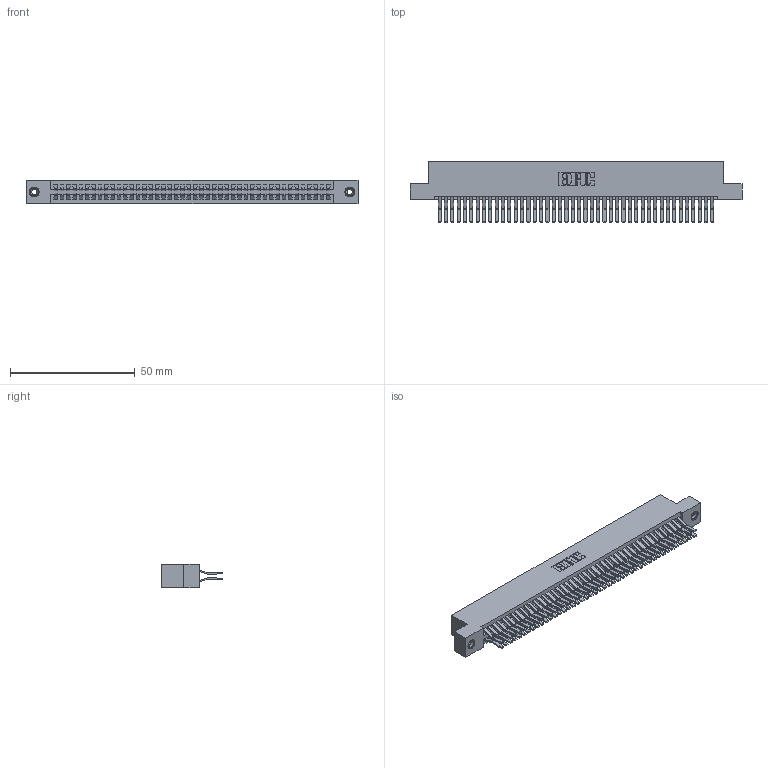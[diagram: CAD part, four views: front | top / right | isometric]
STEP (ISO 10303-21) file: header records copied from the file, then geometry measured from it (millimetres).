
FILE_DESCRIPTION (( 'STEP AP203' ), '1' );
FILE_NAME ('395-088-560-208.STEP', '2019-10-25T15:27:44', ( '' ), ( '' ), 'SwSTEP 2.0', 'SolidWorks 2016', '' );
FILE_SCHEMA (( 'CONFIG_CONTROL_DESIGN' ));
Length unit declared in the file: inch
Products named in the file (4): 345 Part_Flush Mounting Lugs - 0.156 Dia-TI; 345-292-001_560 Tail; 345-250-001_345-250-003-102; 395-088-560-208
Assembly tree (91 placements, depth 2):
  395-088-560-208
    345 Part_Flush Mounting Lugs - 0.156 Dia-TI
    345-292-001_560 Tail  x88
    345-250-001_345-250-003-102  x2
Bounding box: 132.97 x 24.45 x 9.4 mm (x, y, z)
Volume: 13505.6 mm3; surface area: 21499.2 mm2
Topology: 91 solids, 91 shells, 4762 faces, 14117 edges, 9286 vertices
Faces by surface type: plane 3016, cylinder 1730, cone 12, torus 4
Entity records: 35528 total; most frequent: CARTESIAN_POINT 5935, ORIENTED_EDGE 5862, DIRECTION 5261, EDGE_CURVE 2931, LINE 2599, VECTOR 2599, VERTEX_POINT 1948, AXIS2_PLACEMENT_3D 1331
